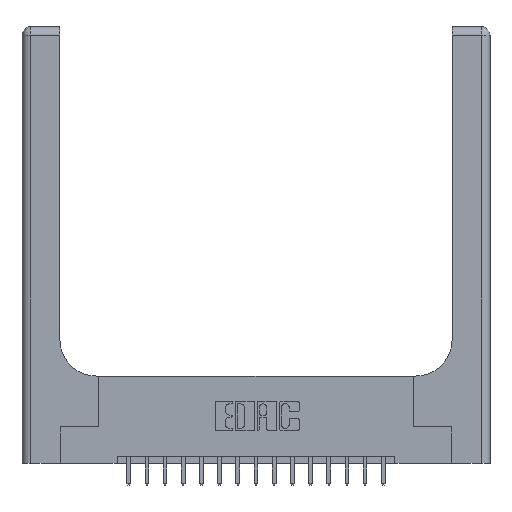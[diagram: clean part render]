
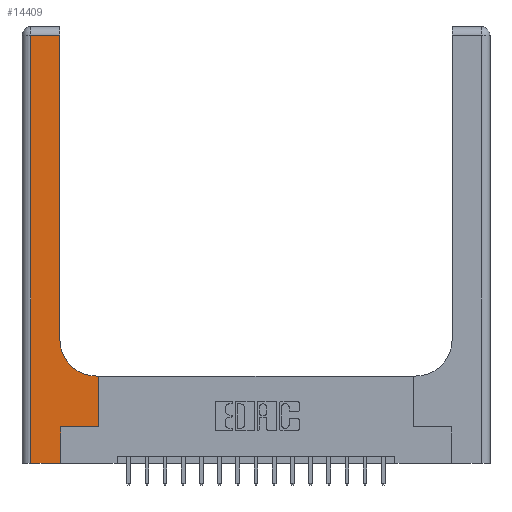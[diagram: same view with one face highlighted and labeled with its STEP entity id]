
A CAD part, top view. The second image highlights one B-rep face of the part: STEP entity #14409.
In plain terms, the highlighted planar face has unit normal (0, 0, 1).
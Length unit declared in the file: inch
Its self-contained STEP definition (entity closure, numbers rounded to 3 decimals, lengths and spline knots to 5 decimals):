
#145 = VERTEX_POINT ( 'NONE', #5000 ) ;
#747 = DIRECTION ( 'NONE',  ( 0., 1., 0. ) ) ;
#847 = LINE ( 'NONE', #18599, #15673 ) ;
#976 = CARTESIAN_POINT ( 'NONE',  ( 0., 2.94, 0.37 ) ) ;
#1967 = ORIENTED_EDGE ( 'NONE', *, *, #17736, .T. ) ;
#2214 = VERTEX_POINT ( 'NONE', #4898 ) ;
#2275 = CARTESIAN_POINT ( 'NONE',  ( 0.265, 0., 0.37 ) ) ;
#2337 = ORIENTED_EDGE ( 'NONE', *, *, #3425, .T. ) ;
#2534 = CARTESIAN_POINT ( 'NONE',  ( 0.265, 0., 0.37 ) ) ;
#2721 = CARTESIAN_POINT ( 'NONE',  ( 0.06, 3., 0.37 ) ) ;
#2893 = FACE_OUTER_BOUND ( 'NONE', #6342, .T. ) ;
#3425 = EDGE_CURVE ( 'NONE', #18147, #145, #14224, .T. ) ;
#3657 = ORIENTED_EDGE ( 'NONE', *, *, #15753, .T. ) ;
#3766 = CARTESIAN_POINT ( 'NONE',  ( 0.51, 0.85, 0.37 ) ) ;
#3793 = EDGE_CURVE ( 'NONE', #15886, #17526, #17650, .T. ) ;
#3813 = DIRECTION ( 'NONE',  ( 0., 1., 0. ) ) ;
#4039 = EDGE_CURVE ( 'NONE', #8587, #15886, #10154, .T. ) ;
#4239 = DIRECTION ( 'NONE',  ( 0., 0., -1. ) ) ;
#4513 = LINE ( 'NONE', #17738, #9520 ) ;
#4802 = LINE ( 'NONE', #9232, #14522 ) ;
#4861 = ORIENTED_EDGE ( 'NONE', *, *, #12401, .T. ) ;
#4898 = CARTESIAN_POINT ( 'NONE',  ( 0.51, 0.6, 0.37 ) ) ;
#5000 = CARTESIAN_POINT ( 'NONE',  ( 0.06, 2.94, 0.37 ) ) ;
#5914 = VECTOR ( 'NONE', #6862, 39.37008 ) ;
#5958 = CARTESIAN_POINT ( 'NONE',  ( 0.265, 0.25, 0.37 ) ) ;
#6342 = EDGE_LOOP ( 'NONE', ( #12931, #2337, #1967, #3657, #11660, #10794, #16244, #13364, #4861 ) ) ;
#6663 = CARTESIAN_POINT ( 'NONE',  ( 0.265, 0.25, 0.37 ) ) ;
#6862 = DIRECTION ( 'NONE',  ( -1., 0., 0. ) ) ;
#7044 = CIRCLE ( 'NONE', #8275, 0.25 ) ;
#7616 = LINE ( 'NONE', #7712, #18202 ) ;
#7712 = CARTESIAN_POINT ( 'NONE',  ( 0., 0., 0.37 ) ) ;
#7828 = CARTESIAN_POINT ( 'NONE',  ( 0.528, 0.6, 0.37 ) ) ;
#8275 = AXIS2_PLACEMENT_3D ( 'NONE', #3766, #4239, #15923 ) ;
#8587 = VERTEX_POINT ( 'NONE', #2534 ) ;
#8593 = DIRECTION ( 'NONE',  ( 0., -1., 0. ) ) ;
#8651 = CARTESIAN_POINT ( 'NONE',  ( 0.26, 0.85, 0.37 ) ) ;
#9232 = CARTESIAN_POINT ( 'NONE',  ( 0.26, 3., 0.37 ) ) ;
#9294 = VECTOR ( 'NONE', #8593, 39.37008 ) ;
#9520 = VECTOR ( 'NONE', #10110, 39.37008 ) ;
#10110 = DIRECTION ( 'NONE',  ( -1., 0., 0. ) ) ;
#10133 = PLANE ( 'NONE',  #15126 ) ;
#10154 = LINE ( 'NONE', #2275, #15265 ) ;
#10235 = CARTESIAN_POINT ( 'NONE',  ( 0.06, 0., 0.37 ) ) ;
#10297 = VERTEX_POINT ( 'NONE', #7828 ) ;
#10447 = CARTESIAN_POINT ( 'NONE',  ( 0.528, 0.25, 0.37 ) ) ;
#10794 = ORIENTED_EDGE ( 'NONE', *, *, #3793, .T. ) ;
#11369 = EDGE_CURVE ( 'NONE', #17526, #10297, #847, .T. ) ;
#11578 = CARTESIAN_POINT ( 'NONE',  ( 0., 3., 0.37 ) ) ;
#11660 = ORIENTED_EDGE ( 'NONE', *, *, #4039, .T. ) ;
#12401 = EDGE_CURVE ( 'NONE', #2214, #13203, #7044, .T. ) ;
#12931 = ORIENTED_EDGE ( 'NONE', *, *, #16317, .T. ) ;
#13150 = EDGE_CURVE ( 'NONE', #10297, #2214, #4513, .T. ) ;
#13203 = VERTEX_POINT ( 'NONE', #8651 ) ;
#13364 = ORIENTED_EDGE ( 'NONE', *, *, #13150, .T. ) ;
#13634 = DIRECTION ( 'NONE',  ( 1., 0., 0. ) ) ;
#14224 = LINE ( 'NONE', #976, #5914 ) ;
#14409 = ADVANCED_FACE ( 'NONE', ( #2893 ), #10133, .F. ) ;
#14522 = VECTOR ( 'NONE', #17847, 39.37008 ) ;
#14684 = DIRECTION ( 'NONE',  ( -1., 0., 0. ) ) ;
#15047 = DIRECTION ( 'NONE',  ( 1., 0., 0. ) ) ;
#15126 = AXIS2_PLACEMENT_3D ( 'NONE', #11578, #18917, #14684 ) ;
#15265 = VECTOR ( 'NONE', #3813, 39.37008 ) ;
#15471 = CARTESIAN_POINT ( 'NONE',  ( 0.26, 2.94, 0.37 ) ) ;
#15673 = VECTOR ( 'NONE', #747, 39.37008 ) ;
#15753 = EDGE_CURVE ( 'NONE', #18024, #8587, #7616, .T. ) ;
#15886 = VERTEX_POINT ( 'NONE', #6663 ) ;
#15923 = DIRECTION ( 'NONE',  ( 1., 0., 0. ) ) ;
#16244 = ORIENTED_EDGE ( 'NONE', *, *, #11369, .T. ) ;
#16317 = EDGE_CURVE ( 'NONE', #13203, #18147, #4802, .T. ) ;
#17526 = VERTEX_POINT ( 'NONE', #10447 ) ;
#17650 = LINE ( 'NONE', #5958, #18307 ) ;
#17736 = EDGE_CURVE ( 'NONE', #145, #18024, #18190, .T. ) ;
#17738 = CARTESIAN_POINT ( 'NONE',  ( 0.26, 0.6, 0.37 ) ) ;
#17847 = DIRECTION ( 'NONE',  ( 0., 1., 0. ) ) ;
#18024 = VERTEX_POINT ( 'NONE', #10235 ) ;
#18147 = VERTEX_POINT ( 'NONE', #15471 ) ;
#18190 = LINE ( 'NONE', #2721, #9294 ) ;
#18202 = VECTOR ( 'NONE', #13634, 39.37008 ) ;
#18307 = VECTOR ( 'NONE', #15047, 39.37008 ) ;
#18599 = CARTESIAN_POINT ( 'NONE',  ( 0.528, 0.25, 0.37 ) ) ;
#18917 = DIRECTION ( 'NONE',  ( 0., 0., -1. ) ) ;
